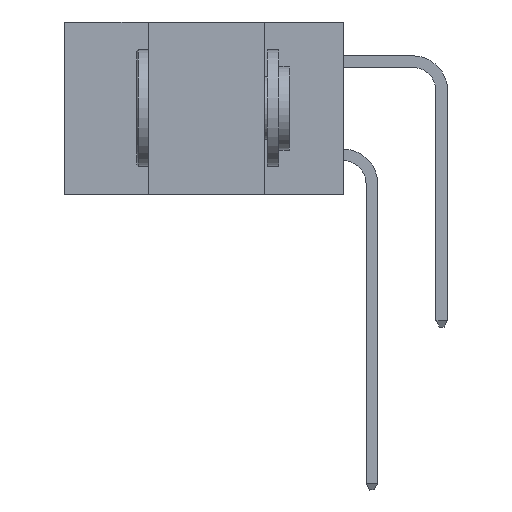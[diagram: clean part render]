
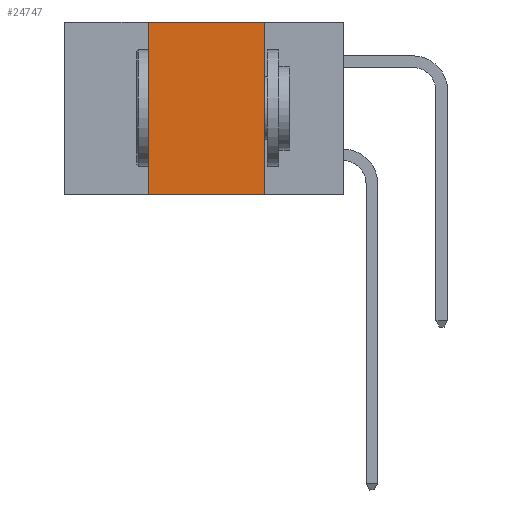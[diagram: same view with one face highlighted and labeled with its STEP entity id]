
A CAD part, left-side view. The second image highlights one B-rep face of the part: STEP entity #24747.
In plain terms, the highlighted planar face has unit normal (-1, 0, 0).
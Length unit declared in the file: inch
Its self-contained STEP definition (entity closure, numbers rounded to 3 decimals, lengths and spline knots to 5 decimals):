
#388 = EDGE_CURVE ( 'NONE', #11969, #20020, #3915, .T. ) ;
#490 = LINE ( 'NONE', #12480, #24365 ) ;
#1351 = ORIENTED_EDGE ( 'NONE', *, *, #5689, .F. ) ;
#1991 = CARTESIAN_POINT ( 'NONE',  ( 0., 0.42, -0.37 ) ) ;
#2861 = CARTESIAN_POINT ( 'NONE',  ( 0., 0.42, 0. ) ) ;
#3013 = CARTESIAN_POINT ( 'NONE',  ( 0., 0.42, -0.37 ) ) ;
#3119 = CARTESIAN_POINT ( 'NONE',  ( 0., 0.17, -0.37 ) ) ;
#3205 = DIRECTION ( 'NONE',  ( 0., 0., -1. ) ) ;
#3502 = DIRECTION ( 'NONE',  ( 0., -1., 0. ) ) ;
#3915 = LINE ( 'NONE', #3013, #18765 ) ;
#4240 = CARTESIAN_POINT ( 'NONE',  ( 0., 0.6, 0. ) ) ;
#4522 = VERTEX_POINT ( 'NONE', #24737 ) ;
#4595 = DIRECTION ( 'NONE',  ( 0., 0., 1. ) ) ;
#4668 = AXIS2_PLACEMENT_3D ( 'NONE', #7032, #10893, #24274 ) ;
#5689 = EDGE_CURVE ( 'NONE', #15838, #4522, #8678, .T. ) ;
#7032 = CARTESIAN_POINT ( 'NONE',  ( 0., 0.6, 0. ) ) ;
#7035 = EDGE_CURVE ( 'NONE', #20020, #15838, #22756, .T. ) ;
#8678 = LINE ( 'NONE', #3119, #14048 ) ;
#10564 = ORIENTED_EDGE ( 'NONE', *, *, #388, .F. ) ;
#10893 = DIRECTION ( 'NONE',  ( 1., 0., 0. ) ) ;
#10895 = EDGE_CURVE ( 'NONE', #11969, #4522, #490, .T. ) ;
#11618 = FACE_OUTER_BOUND ( 'NONE', #19612, .T. ) ;
#11969 = VERTEX_POINT ( 'NONE', #1991 ) ;
#12480 = CARTESIAN_POINT ( 'NONE',  ( 0., 0.6, -0.37 ) ) ;
#12756 = PLANE ( 'NONE',  #4668 ) ;
#14048 = VECTOR ( 'NONE', #3205, 39.37008 ) ;
#14151 = CARTESIAN_POINT ( 'NONE',  ( 0., 0.17, 0. ) ) ;
#15838 = VERTEX_POINT ( 'NONE', #14151 ) ;
#16508 = VECTOR ( 'NONE', #3502, 39.37008 ) ;
#18765 = VECTOR ( 'NONE', #4595, 39.37008 ) ;
#19612 = EDGE_LOOP ( 'NONE', ( #1351, #21357, #10564, #21339 ) ) ;
#20020 = VERTEX_POINT ( 'NONE', #2861 ) ;
#21339 = ORIENTED_EDGE ( 'NONE', *, *, #10895, .T. ) ;
#21357 = ORIENTED_EDGE ( 'NONE', *, *, #7035, .F. ) ;
#21992 = DIRECTION ( 'NONE',  ( 0., -1., 0. ) ) ;
#22756 = LINE ( 'NONE', #4240, #16508 ) ;
#24274 = DIRECTION ( 'NONE',  ( 0., 0., -1. ) ) ;
#24365 = VECTOR ( 'NONE', #21992, 39.37008 ) ;
#24737 = CARTESIAN_POINT ( 'NONE',  ( 0., 0.17, -0.37 ) ) ;
#24747 = ADVANCED_FACE ( 'NONE', ( #11618 ), #12756, .F. ) ;
